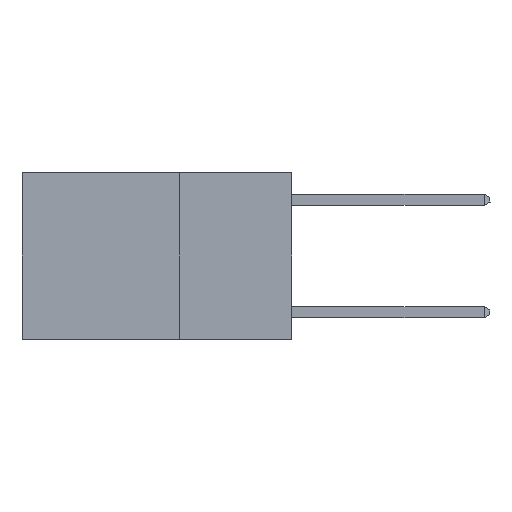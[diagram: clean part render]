
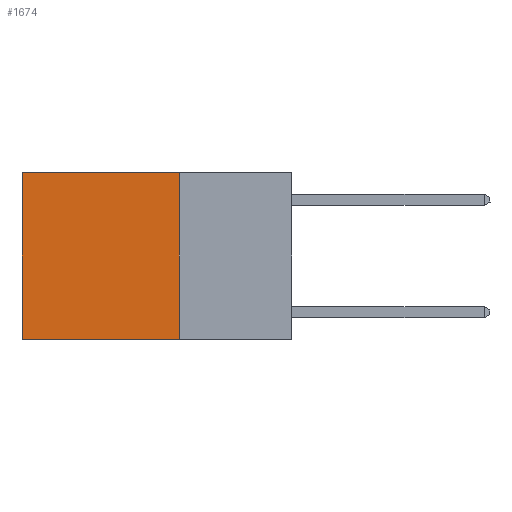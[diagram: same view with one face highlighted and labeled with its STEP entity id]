
A CAD part, left-side view. The second image highlights one B-rep face of the part: STEP entity #1674.
In plain terms, the highlighted planar face has unit normal (-1, 0, 0).
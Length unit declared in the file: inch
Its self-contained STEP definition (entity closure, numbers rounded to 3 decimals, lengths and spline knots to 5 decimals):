
#260 = DIRECTION ( 'NONE',  ( 1., 0., 0. ) ) ;
#357 = EDGE_CURVE ( 'NONE', #26248, #8407, #7451, .T. ) ;
#1485 = ORIENTED_EDGE ( 'NONE', *, *, #19992, .T. ) ;
#1674 = ADVANCED_FACE ( 'NONE', ( #14695 ), #16050, .F. ) ;
#2614 = EDGE_CURVE ( 'NONE', #8407, #25798, #7985, .T. ) ;
#2640 = CARTESIAN_POINT ( 'NONE',  ( 0.2625, 0.25, 0. ) ) ;
#4190 = ORIENTED_EDGE ( 'NONE', *, *, #357, .F. ) ;
#6367 = VECTOR ( 'NONE', #6720, 39.37008 ) ;
#6476 = CARTESIAN_POINT ( 'NONE',  ( 0.2625, 0.25, -0.37 ) ) ;
#6720 = DIRECTION ( 'NONE',  ( 0., 0., -1. ) ) ;
#6862 = DIRECTION ( 'NONE',  ( 0., 1., 0. ) ) ;
#7292 = VECTOR ( 'NONE', #6862, 39.37008 ) ;
#7451 = LINE ( 'NONE', #20979, #6367 ) ;
#7985 = LINE ( 'NONE', #6476, #7292 ) ;
#8214 = CARTESIAN_POINT ( 'NONE',  ( 0.2625, 0.25, -0.37 ) ) ;
#8407 = VERTEX_POINT ( 'NONE', #8214 ) ;
#8780 = LINE ( 'NONE', #17212, #26041 ) ;
#9089 = CARTESIAN_POINT ( 'NONE',  ( 0.2625, 0.25, 0. ) ) ;
#9282 = EDGE_LOOP ( 'NONE', ( #1485, #11424, #4190, #20355 ) ) ;
#10104 = CARTESIAN_POINT ( 'NONE',  ( 0.2625, 0.6, -0.37 ) ) ;
#11424 = ORIENTED_EDGE ( 'NONE', *, *, #2614, .F. ) ;
#14695 = FACE_OUTER_BOUND ( 'NONE', #9282, .T. ) ;
#14884 = AXIS2_PLACEMENT_3D ( 'NONE', #2640, #260, #22965 ) ;
#16050 = PLANE ( 'NONE',  #14884 ) ;
#16333 = DIRECTION ( 'NONE',  ( 0., 0., -1. ) ) ;
#17212 = CARTESIAN_POINT ( 'NONE',  ( 0.2625, 0.25, 0. ) ) ;
#17893 = DIRECTION ( 'NONE',  ( 0., 1., 0. ) ) ;
#19384 = VERTEX_POINT ( 'NONE', #23077 ) ;
#19479 = VECTOR ( 'NONE', #16333, 39.37008 ) ;
#19992 = EDGE_CURVE ( 'NONE', #19384, #25798, #25476, .T. ) ;
#20355 = ORIENTED_EDGE ( 'NONE', *, *, #26607, .T. ) ;
#20979 = CARTESIAN_POINT ( 'NONE',  ( 0.2625, 0.25, 0. ) ) ;
#22965 = DIRECTION ( 'NONE',  ( 0., 0., -1. ) ) ;
#23040 = CARTESIAN_POINT ( 'NONE',  ( 0.2625, 0.6, 0. ) ) ;
#23077 = CARTESIAN_POINT ( 'NONE',  ( 0.2625, 0.6, 0. ) ) ;
#25476 = LINE ( 'NONE', #23040, #19479 ) ;
#25798 = VERTEX_POINT ( 'NONE', #10104 ) ;
#26041 = VECTOR ( 'NONE', #17893, 39.37008 ) ;
#26248 = VERTEX_POINT ( 'NONE', #9089 ) ;
#26607 = EDGE_CURVE ( 'NONE', #26248, #19384, #8780, .T. ) ;
